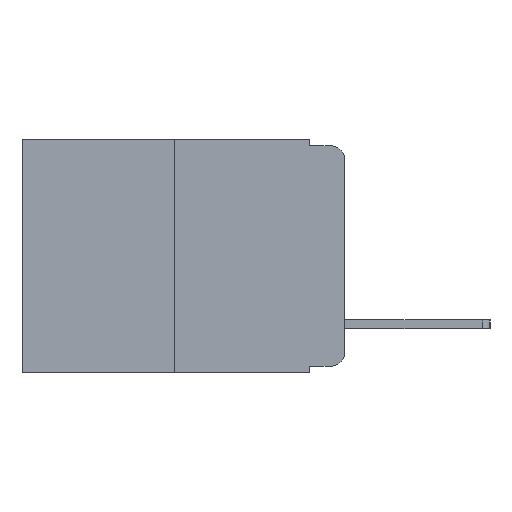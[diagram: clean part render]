
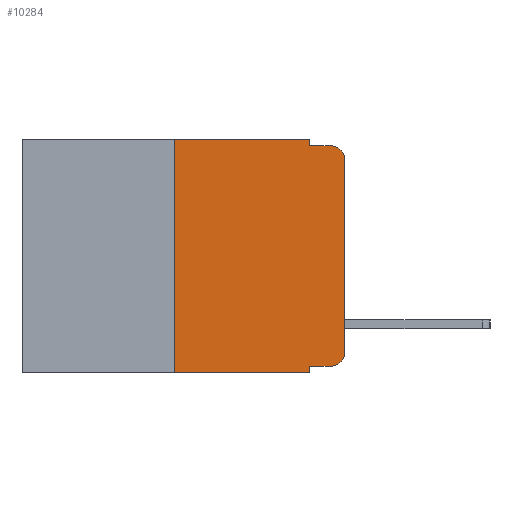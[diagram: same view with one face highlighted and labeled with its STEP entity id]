
A CAD part, left-side view. The second image highlights one B-rep face of the part: STEP entity #10284.
In plain terms, the highlighted planar face has unit normal (-1, 0, 0).
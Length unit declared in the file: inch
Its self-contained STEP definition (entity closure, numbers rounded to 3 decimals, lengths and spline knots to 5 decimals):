
#322 = ORIENTED_EDGE ( 'NONE', *, *, #12249, .F. ) ;
#405 = CARTESIAN_POINT ( 'NONE',  ( 0., 0.051, -0.01 ) ) ;
#452 = CARTESIAN_POINT ( 'NONE',  ( 0., 0.02, -0.333 ) ) ;
#1676 = ORIENTED_EDGE ( 'NONE', *, *, #15737, .T. ) ;
#1919 = CARTESIAN_POINT ( 'NONE',  ( 0., 0.051, 0. ) ) ;
#2112 = EDGE_LOOP ( 'NONE', ( #17629, #1676, #2769, #15171, #19469, #8066, #12654, #322, #5864, #2516 ) ) ;
#2232 = LINE ( 'NONE', #4252, #18102 ) ;
#2516 = ORIENTED_EDGE ( 'NONE', *, *, #13170, .T. ) ;
#2613 = LINE ( 'NONE', #19014, #6449 ) ;
#2769 = ORIENTED_EDGE ( 'NONE', *, *, #7653, .F. ) ;
#3436 = VECTOR ( 'NONE', #16124, 39.37008 ) ;
#3587 = CARTESIAN_POINT ( 'NONE',  ( 0., 0.473, 0. ) ) ;
#3778 = VERTEX_POINT ( 'NONE', #19518 ) ;
#3895 = DIRECTION ( 'NONE',  ( 0., 0., -1. ) ) ;
#4252 = CARTESIAN_POINT ( 'NONE',  ( 0., 0.473, -0.343 ) ) ;
#4743 = CARTESIAN_POINT ( 'NONE',  ( 0., 0.02, -0.01 ) ) ;
#4854 = CARTESIAN_POINT ( 'NONE',  ( 0., 0.25, -0.343 ) ) ;
#5044 = VERTEX_POINT ( 'NONE', #18940 ) ;
#5057 = AXIS2_PLACEMENT_3D ( 'NONE', #16270, #7267, #17718 ) ;
#5398 = EDGE_CURVE ( 'NONE', #14972, #5434, #11739, .T. ) ;
#5429 = FACE_OUTER_BOUND ( 'NONE', #2112, .T. ) ;
#5434 = VERTEX_POINT ( 'NONE', #6694 ) ;
#5577 = LINE ( 'NONE', #17571, #18529 ) ;
#5864 = ORIENTED_EDGE ( 'NONE', *, *, #7495, .T. ) ;
#6449 = VECTOR ( 'NONE', #3895, 39.37008 ) ;
#6519 = VERTEX_POINT ( 'NONE', #452 ) ;
#6681 = CARTESIAN_POINT ( 'NONE',  ( 0., 0.051, -0.333 ) ) ;
#6694 = CARTESIAN_POINT ( 'NONE',  ( 0., 0., -0.03 ) ) ;
#6866 = PLANE ( 'NONE',  #11998 ) ;
#7267 = DIRECTION ( 'NONE',  ( -1., 0., 0. ) ) ;
#7432 = VERTEX_POINT ( 'NONE', #4854 ) ;
#7495 = EDGE_CURVE ( 'NONE', #7952, #6519, #15541, .T. ) ;
#7653 = EDGE_CURVE ( 'NONE', #13417, #17190, #7743, .T. ) ;
#7743 = LINE ( 'NONE', #405, #3436 ) ;
#7952 = VERTEX_POINT ( 'NONE', #10811 ) ;
#8066 = ORIENTED_EDGE ( 'NONE', *, *, #18130, .F. ) ;
#8110 = CIRCLE ( 'NONE', #5057, 0.02 ) ;
#8654 = DIRECTION ( 'NONE',  ( 0., 0., -1. ) ) ;
#9273 = CARTESIAN_POINT ( 'NONE',  ( 0., 0.02, -0.313 ) ) ;
#9781 = EDGE_CURVE ( 'NONE', #14228, #13417, #2613, .T. ) ;
#9930 = DIRECTION ( 'NONE',  ( 0., 0., -1. ) ) ;
#10284 = ADVANCED_FACE ( 'NONE', ( #5429 ), #6866, .F. ) ;
#10792 = DIRECTION ( 'NONE',  ( 0., 0., -1. ) ) ;
#10811 = CARTESIAN_POINT ( 'NONE',  ( 0., 0.051, -0.333 ) ) ;
#10858 = LINE ( 'NONE', #19940, #11354 ) ;
#11246 = CARTESIAN_POINT ( 'NONE',  ( 0., 0., 0. ) ) ;
#11354 = VECTOR ( 'NONE', #12712, 39.37008 ) ;
#11739 = LINE ( 'NONE', #11246, #15706 ) ;
#11998 = AXIS2_PLACEMENT_3D ( 'NONE', #3587, #18818, #9930 ) ;
#12249 = EDGE_CURVE ( 'NONE', #7952, #5044, #5577, .T. ) ;
#12654 = ORIENTED_EDGE ( 'NONE', *, *, #16945, .T. ) ;
#12712 = DIRECTION ( 'NONE',  ( 0., 0., 1. ) ) ;
#12815 = CIRCLE ( 'NONE', #19059, 0.02 ) ;
#13170 = EDGE_CURVE ( 'NONE', #6519, #14972, #12815, .T. ) ;
#13400 = VECTOR ( 'NONE', #14946, 39.37008 ) ;
#13417 = VERTEX_POINT ( 'NONE', #18615 ) ;
#13418 = CARTESIAN_POINT ( 'NONE',  ( 0., 0., -0.313 ) ) ;
#14228 = VERTEX_POINT ( 'NONE', #1919 ) ;
#14946 = DIRECTION ( 'NONE',  ( 0., -1., 0. ) ) ;
#14972 = VERTEX_POINT ( 'NONE', #13418 ) ;
#15171 = ORIENTED_EDGE ( 'NONE', *, *, #9781, .F. ) ;
#15541 = LINE ( 'NONE', #6681, #18467 ) ;
#15706 = VECTOR ( 'NONE', #18607, 39.37008 ) ;
#15737 = EDGE_CURVE ( 'NONE', #5434, #17190, #8110, .T. ) ;
#16124 = DIRECTION ( 'NONE',  ( 0., -1., 0. ) ) ;
#16270 = CARTESIAN_POINT ( 'NONE',  ( 0., 0.02, -0.03 ) ) ;
#16466 = EDGE_CURVE ( 'NONE', #3778, #14228, #17191, .T. ) ;
#16484 = DIRECTION ( 'NONE',  ( 0., -1., 0. ) ) ;
#16945 = EDGE_CURVE ( 'NONE', #7432, #5044, #2232, .T. ) ;
#17189 = DIRECTION ( 'NONE',  ( 0., -1., 0. ) ) ;
#17190 = VERTEX_POINT ( 'NONE', #4743 ) ;
#17191 = LINE ( 'NONE', #19160, #13400 ) ;
#17571 = CARTESIAN_POINT ( 'NONE',  ( 0., 0.051, 0. ) ) ;
#17629 = ORIENTED_EDGE ( 'NONE', *, *, #5398, .T. ) ;
#17718 = DIRECTION ( 'NONE',  ( 0., 0., -1. ) ) ;
#18102 = VECTOR ( 'NONE', #16484, 39.37008 ) ;
#18130 = EDGE_CURVE ( 'NONE', #7432, #3778, #10858, .T. ) ;
#18467 = VECTOR ( 'NONE', #17189, 39.37008 ) ;
#18529 = VECTOR ( 'NONE', #8654, 39.37008 ) ;
#18607 = DIRECTION ( 'NONE',  ( 0., 0., 1. ) ) ;
#18615 = CARTESIAN_POINT ( 'NONE',  ( 0., 0.051, -0.01 ) ) ;
#18818 = DIRECTION ( 'NONE',  ( 1., 0., 0. ) ) ;
#18940 = CARTESIAN_POINT ( 'NONE',  ( 0., 0.051, -0.343 ) ) ;
#19014 = CARTESIAN_POINT ( 'NONE',  ( 0., 0.051, 0. ) ) ;
#19059 = AXIS2_PLACEMENT_3D ( 'NONE', #9273, #19644, #10792 ) ;
#19160 = CARTESIAN_POINT ( 'NONE',  ( 0., 0.473, 0. ) ) ;
#19469 = ORIENTED_EDGE ( 'NONE', *, *, #16466, .F. ) ;
#19518 = CARTESIAN_POINT ( 'NONE',  ( 0., 0.25, 0. ) ) ;
#19644 = DIRECTION ( 'NONE',  ( -1., 0., 0. ) ) ;
#19940 = CARTESIAN_POINT ( 'NONE',  ( 0., 0.25, 0. ) ) ;
